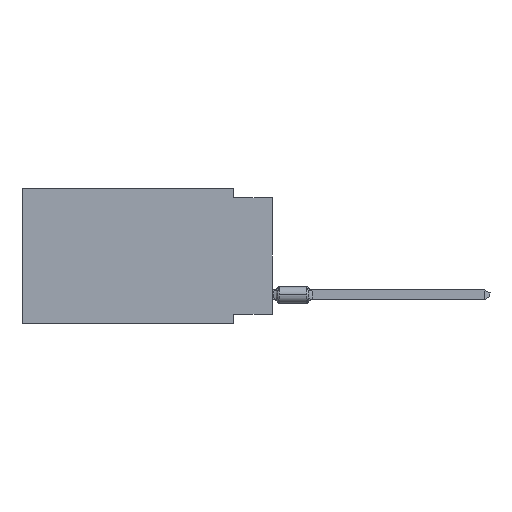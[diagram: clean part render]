
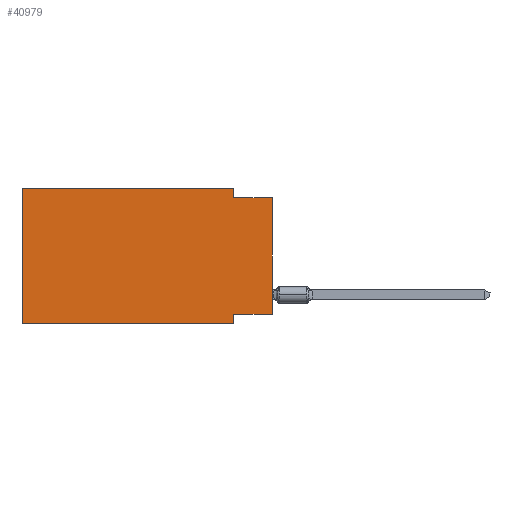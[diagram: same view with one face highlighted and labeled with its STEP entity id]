
A CAD part, left-side view. The second image highlights one B-rep face of the part: STEP entity #40979.
In plain terms, the highlighted planar face has unit normal (-1, 0, 0).
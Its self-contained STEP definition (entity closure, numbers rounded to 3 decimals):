
#600 = VECTOR ( 'NONE', #50017, 1000. ) ;
#1124 = CARTESIAN_POINT ( 'NONE',  ( 0., 0., -0.635 ) ) ;
#1951 = VERTEX_POINT ( 'NONE', #7705 ) ;
#3177 = EDGE_CURVE ( 'NONE', #43533, #25508, #52770, .T. ) ;
#4061 = CARTESIAN_POINT ( 'NONE',  ( 0., 0., -8.255 ) ) ;
#4629 = ORIENTED_EDGE ( 'NONE', *, *, #52240, .T. ) ;
#5469 = CARTESIAN_POINT ( 'NONE',  ( 0., 2.54, 0. ) ) ;
#5617 = ORIENTED_EDGE ( 'NONE', *, *, #49012, .T. ) ;
#7705 = CARTESIAN_POINT ( 'NONE',  ( 0., 2.54, 0. ) ) ;
#8350 = ORIENTED_EDGE ( 'NONE', *, *, #55406, .F. ) ;
#9766 = VECTOR ( 'NONE', #13602, 1000. ) ;
#10040 = CARTESIAN_POINT ( 'NONE',  ( 0., 0., -8.255 ) ) ;
#10356 = LINE ( 'NONE', #27715, #51204 ) ;
#12614 = DIRECTION ( 'NONE',  ( 0., 0., -1. ) ) ;
#12914 = DIRECTION ( 'NONE',  ( 0., -1., 0. ) ) ;
#13602 = DIRECTION ( 'NONE',  ( 0., 1., 0. ) ) ;
#14708 = LINE ( 'NONE', #5469, #600 ) ;
#15520 = VERTEX_POINT ( 'NONE', #50199 ) ;
#16496 = CARTESIAN_POINT ( 'NONE',  ( 0., 2.54, -8.89 ) ) ;
#17318 = ORIENTED_EDGE ( 'NONE', *, *, #3177, .F. ) ;
#18252 = VECTOR ( 'NONE', #49752, 1000. ) ;
#19291 = VERTEX_POINT ( 'NONE', #53105 ) ;
#20066 = ORIENTED_EDGE ( 'NONE', *, *, #57240, .F. ) ;
#21628 = ORIENTED_EDGE ( 'NONE', *, *, #35913, .F. ) ;
#21798 = CARTESIAN_POINT ( 'NONE',  ( 0., 2.54, -8.255 ) ) ;
#22412 = VERTEX_POINT ( 'NONE', #52097 ) ;
#25072 = AXIS2_PLACEMENT_3D ( 'NONE', #30558, #34611, #12614 ) ;
#25508 = VERTEX_POINT ( 'NONE', #16496 ) ;
#25891 = ORIENTED_EDGE ( 'NONE', *, *, #33491, .F. ) ;
#26228 = CARTESIAN_POINT ( 'NONE',  ( 0., 0., 0. ) ) ;
#26798 = DIRECTION ( 'NONE',  ( 0., 0., 1. ) ) ;
#27462 = LINE ( 'NONE', #1124, #18252 ) ;
#27715 = CARTESIAN_POINT ( 'NONE',  ( 0., 16.383, 0. ) ) ;
#28863 = CARTESIAN_POINT ( 'NONE',  ( 0., 2.54, -0.635 ) ) ;
#28983 = VERTEX_POINT ( 'NONE', #10040 ) ;
#30311 = LINE ( 'NONE', #52588, #38699 ) ;
#30419 = LINE ( 'NONE', #4061, #9766 ) ;
#30558 = CARTESIAN_POINT ( 'NONE',  ( 0., 16.383, 0. ) ) ;
#33491 = EDGE_CURVE ( 'NONE', #1951, #39277, #14708, .T. ) ;
#33521 = VECTOR ( 'NONE', #26798, 1000. ) ;
#34611 = DIRECTION ( 'NONE',  ( 1., 0., 0. ) ) ;
#34657 = EDGE_CURVE ( 'NONE', #39277, #19291, #27462, .T. ) ;
#35913 = EDGE_CURVE ( 'NONE', #22412, #1951, #30311, .T. ) ;
#35982 = CARTESIAN_POINT ( 'NONE',  ( 0., 2.54, -8.89 ) ) ;
#38680 = PLANE ( 'NONE',  #25072 ) ;
#38699 = VECTOR ( 'NONE', #48521, 1000. ) ;
#39277 = VERTEX_POINT ( 'NONE', #28863 ) ;
#40384 = VECTOR ( 'NONE', #12914, 1000. ) ;
#40617 = DIRECTION ( 'NONE',  ( 0., 0., -1. ) ) ;
#40979 = ADVANCED_FACE ( 'NONE', ( #52843 ), #38680, .F. ) ;
#43533 = VERTEX_POINT ( 'NONE', #21798 ) ;
#48521 = DIRECTION ( 'NONE',  ( 0., -1., 0. ) ) ;
#48799 = LINE ( 'NONE', #26228, #33521 ) ;
#49012 = EDGE_CURVE ( 'NONE', #15520, #25508, #56915, .T. ) ;
#49752 = DIRECTION ( 'NONE',  ( 0., -1., 0. ) ) ;
#49994 = DIRECTION ( 'NONE',  ( 0., 0., 1. ) ) ;
#50017 = DIRECTION ( 'NONE',  ( 0., 0., -1. ) ) ;
#50199 = CARTESIAN_POINT ( 'NONE',  ( 0., 16.383, -8.89 ) ) ;
#51204 = VECTOR ( 'NONE', #49994, 1000. ) ;
#52097 = CARTESIAN_POINT ( 'NONE',  ( 0., 16.383, 0. ) ) ;
#52240 = EDGE_CURVE ( 'NONE', #28983, #19291, #48799, .T. ) ;
#52488 = VECTOR ( 'NONE', #40617, 1000. ) ;
#52576 = CARTESIAN_POINT ( 'NONE',  ( 0., 16.383, -8.89 ) ) ;
#52588 = CARTESIAN_POINT ( 'NONE',  ( 0., 16.383, 0. ) ) ;
#52770 = LINE ( 'NONE', #35982, #52488 ) ;
#52843 = FACE_OUTER_BOUND ( 'NONE', #54307, .T. ) ;
#53105 = CARTESIAN_POINT ( 'NONE',  ( 0., 0., -0.635 ) ) ;
#54307 = EDGE_LOOP ( 'NONE', ( #4629, #56057, #25891, #21628, #20066, #5617, #17318, #8350 ) ) ;
#55406 = EDGE_CURVE ( 'NONE', #28983, #43533, #30419, .T. ) ;
#56057 = ORIENTED_EDGE ( 'NONE', *, *, #34657, .F. ) ;
#56915 = LINE ( 'NONE', #52576, #40384 ) ;
#57240 = EDGE_CURVE ( 'NONE', #15520, #22412, #10356, .T. ) ;
